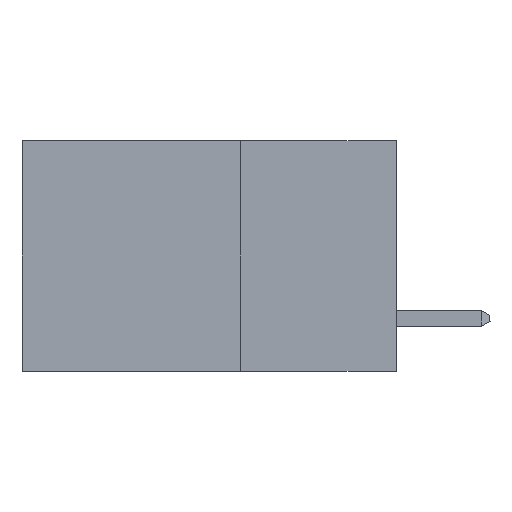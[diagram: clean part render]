
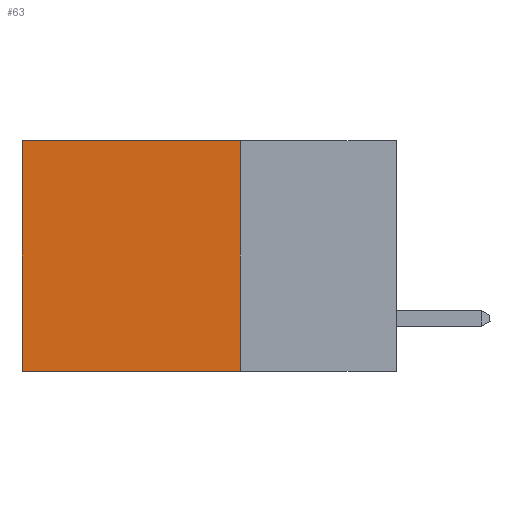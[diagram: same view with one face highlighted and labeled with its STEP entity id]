
A CAD part, left-side view. The second image highlights one B-rep face of the part: STEP entity #63.
In plain terms, the highlighted planar face has unit normal (-1, 0, 0).
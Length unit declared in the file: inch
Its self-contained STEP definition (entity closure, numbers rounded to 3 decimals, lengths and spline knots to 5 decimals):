
#63 = ADVANCED_FACE ( 'NONE', ( #23380 ), #25554, .F. ) ;
#68 = CARTESIAN_POINT ( 'NONE',  ( 0.298, 0.6, 0. ) ) ;
#206 = EDGE_CURVE ( 'NONE', #7613, #28974, #16240, .T. ) ;
#1317 = CARTESIAN_POINT ( 'NONE',  ( 0.298, 0.6, -0.37 ) ) ;
#2160 = VECTOR ( 'NONE', #9174, 39.37008 ) ;
#2804 = ORIENTED_EDGE ( 'NONE', *, *, #20574, .T. ) ;
#3117 = DIRECTION ( 'NONE',  ( 1., 0., 0. ) ) ;
#3451 = CARTESIAN_POINT ( 'NONE',  ( 0.298, 0.6, 0. ) ) ;
#5326 = CARTESIAN_POINT ( 'NONE',  ( 0.298, 0.25, 0. ) ) ;
#5476 = LINE ( 'NONE', #26411, #13648 ) ;
#7142 = CARTESIAN_POINT ( 'NONE',  ( 0.298, 0.25, 0. ) ) ;
#7613 = VERTEX_POINT ( 'NONE', #22236 ) ;
#8086 = VERTEX_POINT ( 'NONE', #1317 ) ;
#8093 = DIRECTION ( 'NONE',  ( 0., 1., 0. ) ) ;
#9174 = DIRECTION ( 'NONE',  ( 0., 0., -1. ) ) ;
#11668 = VECTOR ( 'NONE', #13958, 39.37008 ) ;
#12008 = DIRECTION ( 'NONE',  ( 0., 0., -1. ) ) ;
#12088 = ORIENTED_EDGE ( 'NONE', *, *, #19351, .F. ) ;
#12342 = VERTEX_POINT ( 'NONE', #14610 ) ;
#12807 = ORIENTED_EDGE ( 'NONE', *, *, #27368, .F. ) ;
#13469 = DIRECTION ( 'NONE',  ( 0., 0., -1. ) ) ;
#13648 = VECTOR ( 'NONE', #8093, 39.37008 ) ;
#13958 = DIRECTION ( 'NONE',  ( 0., 1., 0. ) ) ;
#14278 = LINE ( 'NONE', #68, #2160 ) ;
#14610 = CARTESIAN_POINT ( 'NONE',  ( 0.298, 0.25, -0.37 ) ) ;
#15072 = VECTOR ( 'NONE', #13469, 39.37008 ) ;
#16240 = LINE ( 'NONE', #27226, #11668 ) ;
#18630 = LINE ( 'NONE', #7142, #15072 ) ;
#19351 = EDGE_CURVE ( 'NONE', #12342, #8086, #5476, .T. ) ;
#20574 = EDGE_CURVE ( 'NONE', #28974, #8086, #14278, .T. ) ;
#21439 = AXIS2_PLACEMENT_3D ( 'NONE', #5326, #3117, #12008 ) ;
#21517 = EDGE_LOOP ( 'NONE', ( #2804, #12088, #12807, #26466 ) ) ;
#22236 = CARTESIAN_POINT ( 'NONE',  ( 0.298, 0.25, 0. ) ) ;
#23380 = FACE_OUTER_BOUND ( 'NONE', #21517, .T. ) ;
#25554 = PLANE ( 'NONE',  #21439 ) ;
#26411 = CARTESIAN_POINT ( 'NONE',  ( 0.298, 0.25, -0.37 ) ) ;
#26466 = ORIENTED_EDGE ( 'NONE', *, *, #206, .T. ) ;
#27226 = CARTESIAN_POINT ( 'NONE',  ( 0.298, 0.25, 0. ) ) ;
#27368 = EDGE_CURVE ( 'NONE', #7613, #12342, #18630, .T. ) ;
#28974 = VERTEX_POINT ( 'NONE', #3451 ) ;
